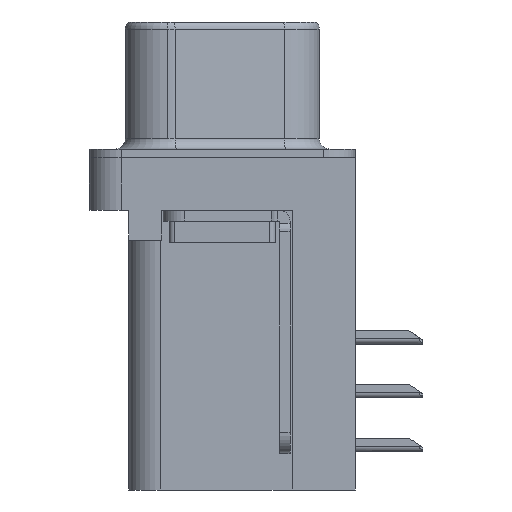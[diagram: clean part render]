
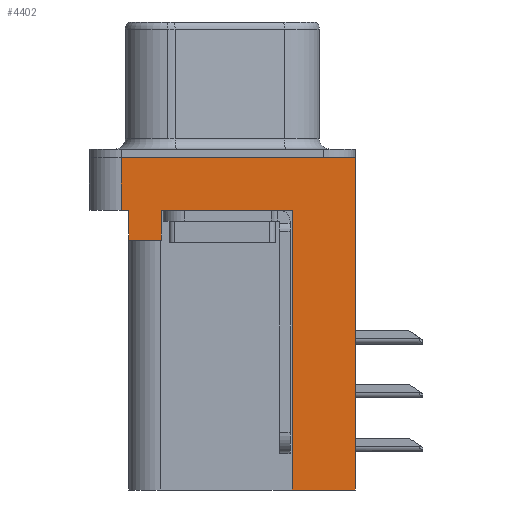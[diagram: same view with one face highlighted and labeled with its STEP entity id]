
A CAD part, left-side view. The second image highlights one B-rep face of the part: STEP entity #4402.
In plain terms, the highlighted planar face has unit normal (-1, 0, 0).
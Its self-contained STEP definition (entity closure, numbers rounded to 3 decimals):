
#119 = ORIENTED_EDGE ( 'NONE', *, *, #22823, .T. ) ;
#155 = DIRECTION ( 'NONE',  ( 0., -1., 0. ) ) ;
#1840 = LINE ( 'NONE', #13005, #20215 ) ;
#2370 = LINE ( 'NONE', #17898, #16363 ) ;
#3173 = ORIENTED_EDGE ( 'NONE', *, *, #5529, .F. ) ;
#3543 = CARTESIAN_POINT ( 'NONE',  ( -2.935, -3.295, -2.5 ) ) ;
#3669 = VECTOR ( 'NONE', #4340, 1000. ) ;
#3733 = LINE ( 'NONE', #13028, #17742 ) ;
#3749 = VERTEX_POINT ( 'NONE', #17073 ) ;
#3960 = LINE ( 'NONE', #12936, #14760 ) ;
#4340 = DIRECTION ( 'NONE',  ( 0., -1., 0. ) ) ;
#4402 = ADVANCED_FACE ( 'NONE', ( #5562 ), #9789, .T. ) ;
#4603 = DIRECTION ( 'NONE',  ( 0., 0., 1. ) ) ;
#4832 = ORIENTED_EDGE ( 'NONE', *, *, #13396, .T. ) ;
#5007 = CARTESIAN_POINT ( 'NONE',  ( -2.935, -3.295, -15.7 ) ) ;
#5134 = CARTESIAN_POINT ( 'NONE',  ( -2.935, 2.895, -3.9 ) ) ;
#5142 = ORIENTED_EDGE ( 'NONE', *, *, #12568, .F. ) ;
#5529 = EDGE_CURVE ( 'NONE', #6336, #17036, #2370, .T. ) ;
#5562 = FACE_OUTER_BOUND ( 'NONE', #22029, .T. ) ;
#6226 = AXIS2_PLACEMENT_3D ( 'NONE', #7929, #22693, #22779 ) ;
#6336 = VERTEX_POINT ( 'NONE', #6779 ) ;
#6779 = CARTESIAN_POINT ( 'NONE',  ( -2.935, -6.275, -15.7 ) ) ;
#7090 = CARTESIAN_POINT ( 'NONE',  ( -2.935, 4.425, -3.9 ) ) ;
#7265 = CARTESIAN_POINT ( 'NONE',  ( -2.935, 4.775, -2.5 ) ) ;
#7929 = CARTESIAN_POINT ( 'NONE',  ( -2.935, -6.275, -2.5 ) ) ;
#8306 = VERTEX_POINT ( 'NONE', #12084 ) ;
#8481 = VECTOR ( 'NONE', #16219, 1000. ) ;
#8781 = EDGE_CURVE ( 'NONE', #17036, #13220, #19046, .T. ) ;
#8908 = VECTOR ( 'NONE', #18815, 1000. ) ;
#9021 = LINE ( 'NONE', #17098, #3669 ) ;
#9178 = ORIENTED_EDGE ( 'NONE', *, *, #20418, .F. ) ;
#9525 = CARTESIAN_POINT ( 'NONE',  ( -2.935, 4.775, 0. ) ) ;
#9789 = PLANE ( 'NONE',  #6226 ) ;
#10553 = EDGE_CURVE ( 'NONE', #13092, #3749, #13509, .T. ) ;
#11504 = LINE ( 'NONE', #17363, #20155 ) ;
#12004 = VERTEX_POINT ( 'NONE', #7265 ) ;
#12084 = CARTESIAN_POINT ( 'NONE',  ( -2.935, -6.275, 0. ) ) ;
#12499 = ORIENTED_EDGE ( 'NONE', *, *, #8781, .F. ) ;
#12568 = EDGE_CURVE ( 'NONE', #13092, #23361, #22698, .T. ) ;
#12936 = CARTESIAN_POINT ( 'NONE',  ( -2.935, -6.275, 0. ) ) ;
#13005 = CARTESIAN_POINT ( 'NONE',  ( -2.935, -6.275, -2.5 ) ) ;
#13028 = CARTESIAN_POINT ( 'NONE',  ( -2.935, -6.275, -2.5 ) ) ;
#13092 = VERTEX_POINT ( 'NONE', #5134 ) ;
#13094 = DIRECTION ( 'NONE',  ( 0., 0., 1. ) ) ;
#13220 = VERTEX_POINT ( 'NONE', #3543 ) ;
#13327 = VERTEX_POINT ( 'NONE', #9525 ) ;
#13396 = EDGE_CURVE ( 'NONE', #12004, #16700, #9021, .T. ) ;
#13509 = LINE ( 'NONE', #14023, #17839 ) ;
#14023 = CARTESIAN_POINT ( 'NONE',  ( -2.935, 2.895, -3.9 ) ) ;
#14143 = VECTOR ( 'NONE', #13094, 1000. ) ;
#14192 = ORIENTED_EDGE ( 'NONE', *, *, #10553, .T. ) ;
#14264 = DIRECTION ( 'NONE',  ( 0., 1., 0. ) ) ;
#14760 = VECTOR ( 'NONE', #155, 1000. ) ;
#14941 = CARTESIAN_POINT ( 'NONE',  ( -2.935, 4.425, -3.9 ) ) ;
#15008 = CARTESIAN_POINT ( 'NONE',  ( -2.935, 4.425, -2.5 ) ) ;
#16219 = DIRECTION ( 'NONE',  ( 0., 1., 0. ) ) ;
#16363 = VECTOR ( 'NONE', #14264, 1000. ) ;
#16700 = VERTEX_POINT ( 'NONE', #15008 ) ;
#16783 = CARTESIAN_POINT ( 'NONE',  ( -2.935, -3.295, -15.7 ) ) ;
#16953 = CARTESIAN_POINT ( 'NONE',  ( -2.935, 4.775, -2.5 ) ) ;
#17036 = VERTEX_POINT ( 'NONE', #5007 ) ;
#17073 = CARTESIAN_POINT ( 'NONE',  ( -2.935, 2.895, -2.5 ) ) ;
#17098 = CARTESIAN_POINT ( 'NONE',  ( -2.935, -6.275, -2.5 ) ) ;
#17266 = EDGE_CURVE ( 'NONE', #13327, #8306, #3960, .T. ) ;
#17363 = CARTESIAN_POINT ( 'NONE',  ( -2.935, 4.425, -3.9 ) ) ;
#17742 = VECTOR ( 'NONE', #18588, 1000. ) ;
#17839 = VECTOR ( 'NONE', #23314, 1000. ) ;
#17898 = CARTESIAN_POINT ( 'NONE',  ( -2.935, -3.295, -15.7 ) ) ;
#17909 = ORIENTED_EDGE ( 'NONE', *, *, #17266, .F. ) ;
#18588 = DIRECTION ( 'NONE',  ( 0., 0., 1. ) ) ;
#18648 = DIRECTION ( 'NONE',  ( 0., -1., 0. ) ) ;
#18803 = EDGE_CURVE ( 'NONE', #3749, #13220, #1840, .T. ) ;
#18815 = DIRECTION ( 'NONE',  ( 0., 0., 1. ) ) ;
#19046 = LINE ( 'NONE', #16783, #14143 ) ;
#20155 = VECTOR ( 'NONE', #4603, 1000. ) ;
#20215 = VECTOR ( 'NONE', #18648, 1000. ) ;
#20271 = ORIENTED_EDGE ( 'NONE', *, *, #18803, .T. ) ;
#20275 = EDGE_CURVE ( 'NONE', #12004, #13327, #23710, .T. ) ;
#20418 = EDGE_CURVE ( 'NONE', #23361, #16700, #11504, .T. ) ;
#21155 = ORIENTED_EDGE ( 'NONE', *, *, #20275, .F. ) ;
#22029 = EDGE_LOOP ( 'NONE', ( #17909, #21155, #4832, #9178, #5142, #14192, #20271, #12499, #3173, #119 ) ) ;
#22693 = DIRECTION ( 'NONE',  ( -1., 0., 0. ) ) ;
#22698 = LINE ( 'NONE', #7090, #8481 ) ;
#22779 = DIRECTION ( 'NONE',  ( 0., 0., 1. ) ) ;
#22823 = EDGE_CURVE ( 'NONE', #6336, #8306, #3733, .T. ) ;
#23314 = DIRECTION ( 'NONE',  ( 0., 0., 1. ) ) ;
#23361 = VERTEX_POINT ( 'NONE', #14941 ) ;
#23710 = LINE ( 'NONE', #16953, #8908 ) ;
